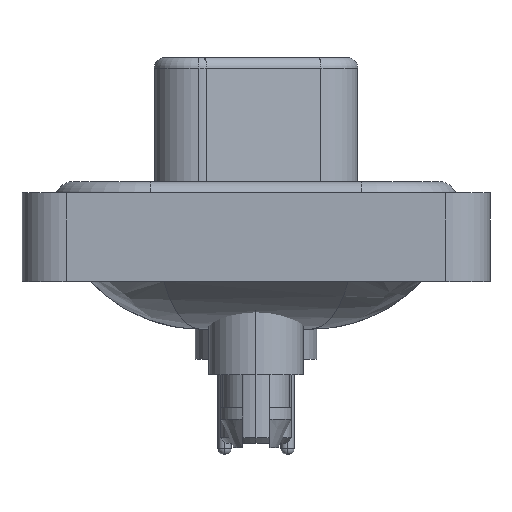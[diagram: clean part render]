
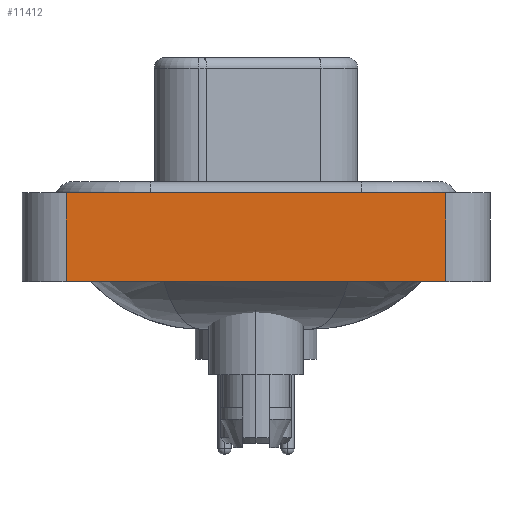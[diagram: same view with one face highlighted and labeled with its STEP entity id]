
A CAD part, left-side view. The second image highlights one B-rep face of the part: STEP entity #11412.
In plain terms, the highlighted planar face has unit normal (-1, 0, 0).
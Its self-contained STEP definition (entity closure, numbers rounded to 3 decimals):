
#1600 = DIRECTION ( 'NONE',  ( -1., 0., 0. ) ) ;
#1721 = DIRECTION ( 'NONE',  ( 0., 0., 1. ) ) ;
#1852 = LINE ( 'NONE', #10503, #18279 ) ;
#1977 = LINE ( 'NONE', #23666, #11946 ) ;
#3537 = ORIENTED_EDGE ( 'NONE', *, *, #14520, .T. ) ;
#3559 = LINE ( 'NONE', #7789, #12793 ) ;
#5490 = VERTEX_POINT ( 'NONE', #24720 ) ;
#7661 = ORIENTED_EDGE ( 'NONE', *, *, #21497, .T. ) ;
#7789 = CARTESIAN_POINT ( 'NONE',  ( -7.35, -8.55, -3.6 ) ) ;
#10308 = ORIENTED_EDGE ( 'NONE', *, *, #24009, .F. ) ;
#10503 = CARTESIAN_POINT ( 'NONE',  ( -7.35, -8.55, -3.6 ) ) ;
#10523 = DIRECTION ( 'NONE',  ( 0., 0., 1. ) ) ;
#10690 = CARTESIAN_POINT ( 'NONE',  ( -7.35, -8.55, 0.4 ) ) ;
#11412 = ADVANCED_FACE ( 'NONE', ( #12948 ), #16771, .T. ) ;
#11946 = VECTOR ( 'NONE', #1721, 1000. ) ;
#12198 = DIRECTION ( 'NONE',  ( 0., 0., 1. ) ) ;
#12793 = VECTOR ( 'NONE', #12198, 1000. ) ;
#12806 = DIRECTION ( 'NONE',  ( 0., -1., 0. ) ) ;
#12948 = FACE_OUTER_BOUND ( 'NONE', #19948, .T. ) ;
#13326 = VECTOR ( 'NONE', #12806, 1000. ) ;
#14421 = VERTEX_POINT ( 'NONE', #16583 ) ;
#14520 = EDGE_CURVE ( 'NONE', #14421, #5490, #3559, .T. ) ;
#14635 = CARTESIAN_POINT ( 'NONE',  ( -7.35, -8.55, -3.6 ) ) ;
#16583 = CARTESIAN_POINT ( 'NONE',  ( -7.35, -8.55, -3.6 ) ) ;
#16771 = PLANE ( 'NONE',  #20281 ) ;
#17567 = CARTESIAN_POINT ( 'NONE',  ( -7.35, 8.55, 0.4 ) ) ;
#18279 = VECTOR ( 'NONE', #19155, 1000. ) ;
#18934 = VERTEX_POINT ( 'NONE', #23528 ) ;
#19155 = DIRECTION ( 'NONE',  ( 0., -1., 0. ) ) ;
#19948 = EDGE_LOOP ( 'NONE', ( #3537, #24628, #10308, #7661 ) ) ;
#20281 = AXIS2_PLACEMENT_3D ( 'NONE', #14635, #1600, #10523 ) ;
#21497 = EDGE_CURVE ( 'NONE', #18934, #14421, #1852, .T. ) ;
#21724 = LINE ( 'NONE', #10690, #13326 ) ;
#23528 = CARTESIAN_POINT ( 'NONE',  ( -7.35, 8.55, -3.6 ) ) ;
#23666 = CARTESIAN_POINT ( 'NONE',  ( -7.35, 8.55, -3.6 ) ) ;
#24009 = EDGE_CURVE ( 'NONE', #18934, #26669, #1977, .T. ) ;
#24628 = ORIENTED_EDGE ( 'NONE', *, *, #24786, .F. ) ;
#24720 = CARTESIAN_POINT ( 'NONE',  ( -7.35, -8.55, 0.4 ) ) ;
#24786 = EDGE_CURVE ( 'NONE', #26669, #5490, #21724, .T. ) ;
#26669 = VERTEX_POINT ( 'NONE', #17567 ) ;
